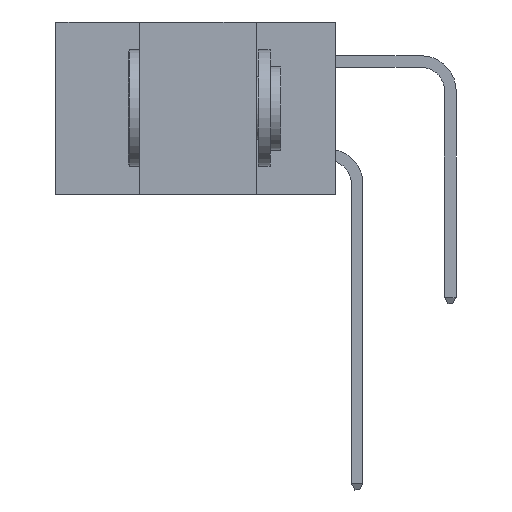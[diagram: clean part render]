
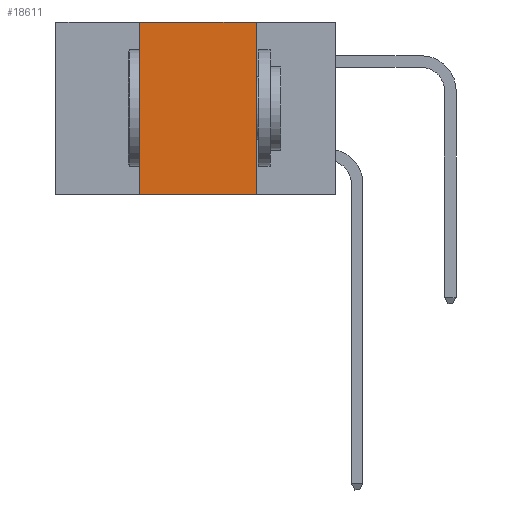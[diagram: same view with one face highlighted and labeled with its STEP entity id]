
A CAD part, left-side view. The second image highlights one B-rep face of the part: STEP entity #18611.
In plain terms, the highlighted planar face has unit normal (-1, 0, 0).
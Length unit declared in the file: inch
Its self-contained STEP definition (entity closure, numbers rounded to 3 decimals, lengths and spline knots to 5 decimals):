
#2261 = ORIENTED_EDGE ( 'NONE', *, *, #25703, .F. ) ;
#2409 = CARTESIAN_POINT ( 'NONE',  ( 0., 0.17, 0. ) ) ;
#4972 = DIRECTION ( 'NONE',  ( 0., -1., 0. ) ) ;
#6879 = LINE ( 'NONE', #14973, #33062 ) ;
#7148 = CARTESIAN_POINT ( 'NONE',  ( 0., 0.42, -0.37 ) ) ;
#7327 = LINE ( 'NONE', #32106, #23124 ) ;
#7382 = CARTESIAN_POINT ( 'NONE',  ( 0., 0.42, 0. ) ) ;
#7606 = CARTESIAN_POINT ( 'NONE',  ( 0., 0.42, 0. ) ) ;
#12361 = CARTESIAN_POINT ( 'NONE',  ( 0., 0.17, 0. ) ) ;
#12958 = LINE ( 'NONE', #12361, #18921 ) ;
#13476 = ORIENTED_EDGE ( 'NONE', *, *, #38552, .F. ) ;
#14057 = AXIS2_PLACEMENT_3D ( 'NONE', #22404, #19361, #22560 ) ;
#14973 = CARTESIAN_POINT ( 'NONE',  ( 0., 0.6, 0. ) ) ;
#16190 = VERTEX_POINT ( 'NONE', #7148 ) ;
#18381 = VERTEX_POINT ( 'NONE', #7382 ) ;
#18611 = ADVANCED_FACE ( 'NONE', ( #34167 ), #33235, .F. ) ;
#18921 = VECTOR ( 'NONE', #29414, 39.37008 ) ;
#19361 = DIRECTION ( 'NONE',  ( 1., 0., 0. ) ) ;
#19537 = VERTEX_POINT ( 'NONE', #35113 ) ;
#19766 = EDGE_CURVE ( 'NONE', #36280, #19537, #12958, .T. ) ;
#22404 = CARTESIAN_POINT ( 'NONE',  ( 0., 0.6, 0. ) ) ;
#22560 = DIRECTION ( 'NONE',  ( 0., 0., -1. ) ) ;
#23124 = VECTOR ( 'NONE', #4972, 39.37008 ) ;
#24817 = EDGE_LOOP ( 'NONE', ( #44627, #2261, #13476, #33538 ) ) ;
#25330 = DIRECTION ( 'NONE',  ( 0., -1., 0. ) ) ;
#25703 = EDGE_CURVE ( 'NONE', #18381, #36280, #6879, .T. ) ;
#29414 = DIRECTION ( 'NONE',  ( 0., 0., -1. ) ) ;
#32106 = CARTESIAN_POINT ( 'NONE',  ( 0., 0.6, -0.37 ) ) ;
#33062 = VECTOR ( 'NONE', #25330, 39.37008 ) ;
#33235 = PLANE ( 'NONE',  #14057 ) ;
#33538 = ORIENTED_EDGE ( 'NONE', *, *, #36119, .T. ) ;
#34167 = FACE_OUTER_BOUND ( 'NONE', #24817, .T. ) ;
#35113 = CARTESIAN_POINT ( 'NONE',  ( 0., 0.17, -0.37 ) ) ;
#36119 = EDGE_CURVE ( 'NONE', #16190, #19537, #7327, .T. ) ;
#36280 = VERTEX_POINT ( 'NONE', #2409 ) ;
#38552 = EDGE_CURVE ( 'NONE', #16190, #18381, #42203, .T. ) ;
#39010 = DIRECTION ( 'NONE',  ( 0., 0., 1. ) ) ;
#41095 = VECTOR ( 'NONE', #39010, 39.37008 ) ;
#42203 = LINE ( 'NONE', #7606, #41095 ) ;
#44627 = ORIENTED_EDGE ( 'NONE', *, *, #19766, .F. ) ;
